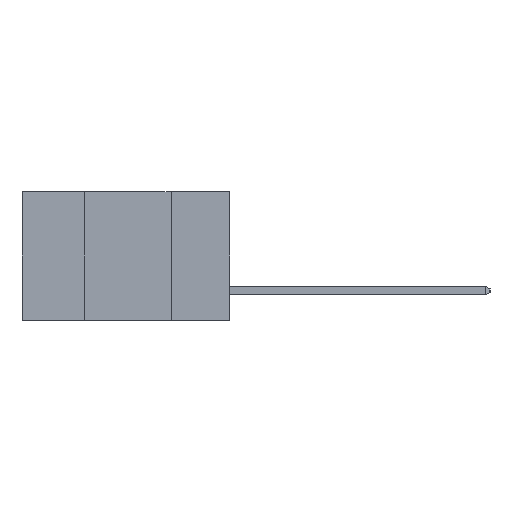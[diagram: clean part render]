
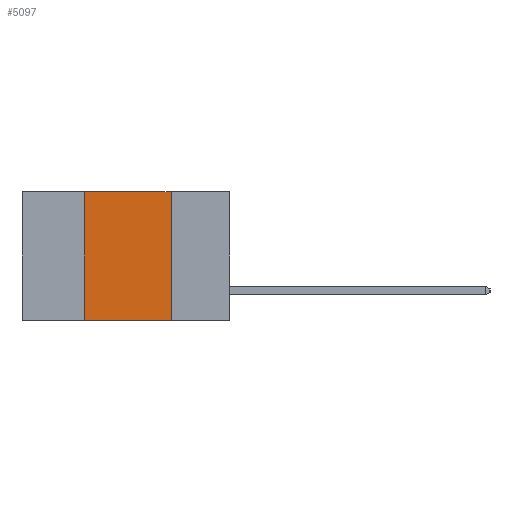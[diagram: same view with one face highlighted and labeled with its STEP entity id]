
A CAD part, left-side view. The second image highlights one B-rep face of the part: STEP entity #5097.
In plain terms, the highlighted planar face has unit normal (-1, 0, 0).
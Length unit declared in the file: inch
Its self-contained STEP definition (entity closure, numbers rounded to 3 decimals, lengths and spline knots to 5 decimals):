
#481 = DIRECTION ( 'NONE',  ( 0., -1., 0. ) ) ;
#869 = VECTOR ( 'NONE', #481, 39.37008 ) ;
#1213 = LINE ( 'NONE', #4647, #10571 ) ;
#1296 = ORIENTED_EDGE ( 'NONE', *, *, #10102, .F. ) ;
#1677 = LINE ( 'NONE', #9960, #10981 ) ;
#1705 = DIRECTION ( 'NONE',  ( 0., 0., -1. ) ) ;
#1767 = VECTOR ( 'NONE', #1705, 39.37008 ) ;
#1789 = DIRECTION ( 'NONE',  ( 0., -1., 0. ) ) ;
#1892 = ORIENTED_EDGE ( 'NONE', *, *, #3332, .F. ) ;
#2371 = CARTESIAN_POINT ( 'NONE',  ( 0., 0.6, -0.37 ) ) ;
#3332 = EDGE_CURVE ( 'NONE', #4714, #7816, #6778, .T. ) ;
#3414 = LINE ( 'NONE', #2371, #869 ) ;
#3547 = ORIENTED_EDGE ( 'NONE', *, *, #11398, .T. ) ;
#3967 = CARTESIAN_POINT ( 'NONE',  ( 0., 0.42, -0.37 ) ) ;
#4595 = EDGE_LOOP ( 'NONE', ( #1892, #1296, #10902, #3547 ) ) ;
#4647 = CARTESIAN_POINT ( 'NONE',  ( 0., 0.6, 0. ) ) ;
#4714 = VERTEX_POINT ( 'NONE', #9912 ) ;
#5097 = ADVANCED_FACE ( 'NONE', ( #11673 ), #5359, .F. ) ;
#5359 = PLANE ( 'NONE',  #9690 ) ;
#5803 = VERTEX_POINT ( 'NONE', #3967 ) ;
#5955 = CARTESIAN_POINT ( 'NONE',  ( 0., 0.17, 0. ) ) ;
#6778 = LINE ( 'NONE', #5955, #1767 ) ;
#7424 = DIRECTION ( 'NONE',  ( 1., 0., 0. ) ) ;
#7773 = CARTESIAN_POINT ( 'NONE',  ( 0., 0.17, -0.37 ) ) ;
#7816 = VERTEX_POINT ( 'NONE', #7773 ) ;
#9100 = VERTEX_POINT ( 'NONE', #9580 ) ;
#9391 = EDGE_CURVE ( 'NONE', #5803, #9100, #1677, .T. ) ;
#9580 = CARTESIAN_POINT ( 'NONE',  ( 0., 0.42, 0. ) ) ;
#9690 = AXIS2_PLACEMENT_3D ( 'NONE', #10793, #7424, #10836 ) ;
#9912 = CARTESIAN_POINT ( 'NONE',  ( 0., 0.17, 0. ) ) ;
#9960 = CARTESIAN_POINT ( 'NONE',  ( 0., 0.42, 0. ) ) ;
#10102 = EDGE_CURVE ( 'NONE', #9100, #4714, #1213, .T. ) ;
#10571 = VECTOR ( 'NONE', #1789, 39.37008 ) ;
#10793 = CARTESIAN_POINT ( 'NONE',  ( 0., 0.6, 0. ) ) ;
#10801 = DIRECTION ( 'NONE',  ( 0., 0., 1. ) ) ;
#10836 = DIRECTION ( 'NONE',  ( 0., 0., -1. ) ) ;
#10902 = ORIENTED_EDGE ( 'NONE', *, *, #9391, .F. ) ;
#10981 = VECTOR ( 'NONE', #10801, 39.37008 ) ;
#11398 = EDGE_CURVE ( 'NONE', #5803, #7816, #3414, .T. ) ;
#11673 = FACE_OUTER_BOUND ( 'NONE', #4595, .T. ) ;
